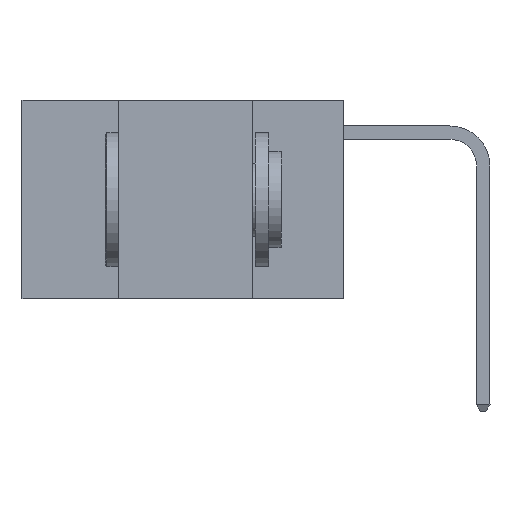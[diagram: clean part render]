
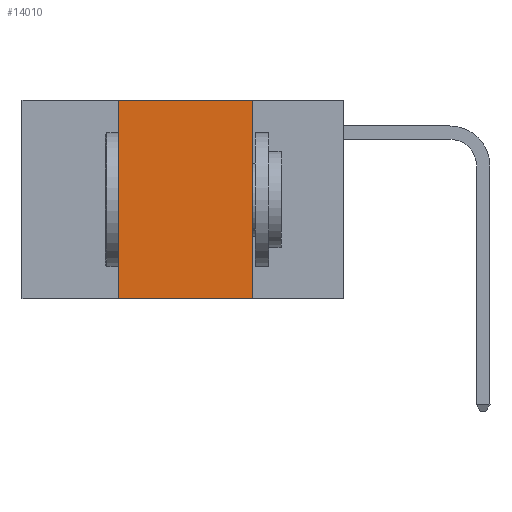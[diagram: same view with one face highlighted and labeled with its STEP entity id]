
A CAD part, left-side view. The second image highlights one B-rep face of the part: STEP entity #14010.
In plain terms, the highlighted planar face has unit normal (-1, 0, 0).
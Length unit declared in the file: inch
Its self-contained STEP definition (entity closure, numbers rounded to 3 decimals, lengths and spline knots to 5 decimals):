
#317 = AXIS2_PLACEMENT_3D ( 'NONE', #15280, #420, #9597 ) ;
#420 = DIRECTION ( 'NONE',  ( 1., 0., 0. ) ) ;
#1065 = VERTEX_POINT ( 'NONE', #14124 ) ;
#2086 = DIRECTION ( 'NONE',  ( 0., -1., 0. ) ) ;
#2195 = VECTOR ( 'NONE', #8509, 39.37008 ) ;
#2499 = ORIENTED_EDGE ( 'NONE', *, *, #12089, .F. ) ;
#3060 = ORIENTED_EDGE ( 'NONE', *, *, #11537, .F. ) ;
#3757 = LINE ( 'NONE', #9671, #2195 ) ;
#3864 = ORIENTED_EDGE ( 'NONE', *, *, #14640, .T. ) ;
#4759 = LINE ( 'NONE', #8087, #15688 ) ;
#5333 = EDGE_CURVE ( 'NONE', #1065, #11046, #3757, .T. ) ;
#6058 = DIRECTION ( 'NONE',  ( 0., -1., 0. ) ) ;
#6122 = DIRECTION ( 'NONE',  ( 0., 0., 1. ) ) ;
#7339 = ORIENTED_EDGE ( 'NONE', *, *, #5333, .F. ) ;
#7370 = CARTESIAN_POINT ( 'NONE',  ( 0., 0.42, 0. ) ) ;
#8068 = FACE_OUTER_BOUND ( 'NONE', #13134, .T. ) ;
#8087 = CARTESIAN_POINT ( 'NONE',  ( 0., 0.6, 0. ) ) ;
#8509 = DIRECTION ( 'NONE',  ( 0., 0., -1. ) ) ;
#8665 = VECTOR ( 'NONE', #6058, 39.37008 ) ;
#9597 = DIRECTION ( 'NONE',  ( 0., 0., -1. ) ) ;
#9671 = CARTESIAN_POINT ( 'NONE',  ( 0., 0.17, 0. ) ) ;
#10126 = VECTOR ( 'NONE', #6122, 39.37008 ) ;
#10427 = LINE ( 'NONE', #16316, #8665 ) ;
#11046 = VERTEX_POINT ( 'NONE', #15039 ) ;
#11537 = EDGE_CURVE ( 'NONE', #17265, #17323, #16479, .T. ) ;
#12089 = EDGE_CURVE ( 'NONE', #17323, #1065, #4759, .T. ) ;
#13134 = EDGE_LOOP ( 'NONE', ( #7339, #2499, #3060, #3864 ) ) ;
#13635 = PLANE ( 'NONE',  #317 ) ;
#14010 = ADVANCED_FACE ( 'NONE', ( #8068 ), #13635, .F. ) ;
#14124 = CARTESIAN_POINT ( 'NONE',  ( 0., 0.17, 0. ) ) ;
#14640 = EDGE_CURVE ( 'NONE', #17265, #11046, #10427, .T. ) ;
#15039 = CARTESIAN_POINT ( 'NONE',  ( 0., 0.17, -0.37 ) ) ;
#15280 = CARTESIAN_POINT ( 'NONE',  ( 0., 0.6, 0. ) ) ;
#15688 = VECTOR ( 'NONE', #2086, 39.37008 ) ;
#16150 = CARTESIAN_POINT ( 'NONE',  ( 0., 0.42, -0.37 ) ) ;
#16316 = CARTESIAN_POINT ( 'NONE',  ( 0., 0.6, -0.37 ) ) ;
#16479 = LINE ( 'NONE', #19099, #10126 ) ;
#17265 = VERTEX_POINT ( 'NONE', #16150 ) ;
#17323 = VERTEX_POINT ( 'NONE', #7370 ) ;
#19099 = CARTESIAN_POINT ( 'NONE',  ( 0., 0.42, 0. ) ) ;
